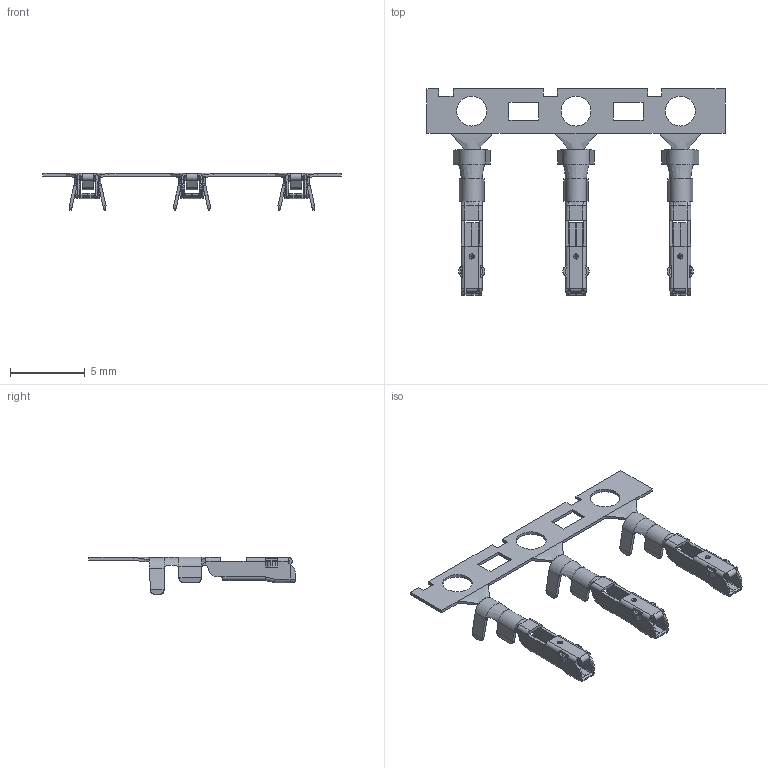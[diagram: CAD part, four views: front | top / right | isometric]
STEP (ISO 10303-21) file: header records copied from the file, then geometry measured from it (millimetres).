
FILE_DESCRIPTION (( 'STEP AP214' ), '1' );
FILE_NAME ('565-290-721 STRIP.STEP', '2020-09-17T17:25:07', ( '' ), ( '' ), 'SwSTEP 2.0', 'SolidWorks 2020', '' );
FILE_SCHEMA (( 'AUTOMOTIVE_DESIGN' ));
Length unit declared in the file: millimetre
Products named in the file (5): 565-290-721-R2-2; 565-292-721-CARRIER-STRIP; 565-290-721-R2-1; 565-290-721-R2-3; 565-290-721 STRIP
Assembly tree (4 placements, depth 2):
  565-290-721 STRIP
    565-292-721-CARRIER-STRIP
    565-290-721-R2-1
    565-290-721-R2-2
    565-290-721-R2-3
Bounding box: 20 x 13.85 x 2.5 mm (x, y, z)
Volume: 33.5 mm3; surface area: 392.9 mm2
Topology: 4 solids, 4 shells, 734 faces, 2028 edges, 1278 vertices
Faces by surface type: plane 350, cylinder 228, bspline 108, torus 18, cone 18, sphere 12
Entity records: 27529 total; most frequent: CARTESIAN_POINT 9533, ORIENTED_EDGE 4056, DIRECTION 3258, EDGE_CURVE 2028, VERTEX_POINT 1278, LINE 1212, VECTOR 1212, AXIS2_PLACEMENT_3D 1023
